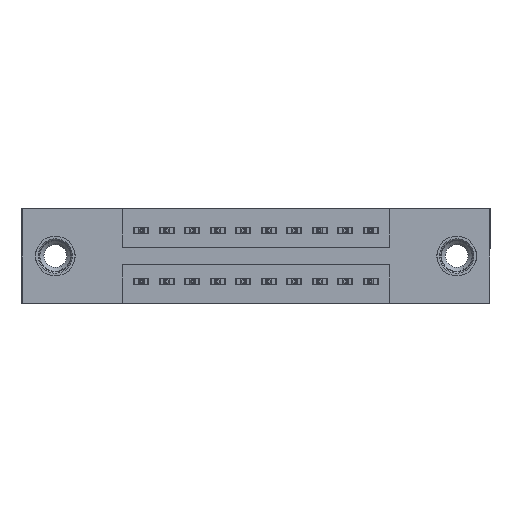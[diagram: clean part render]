
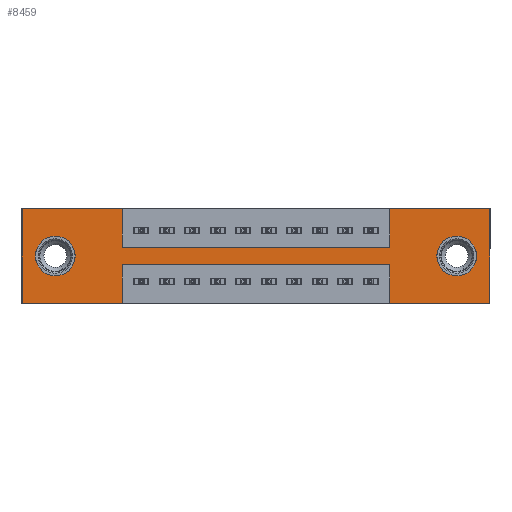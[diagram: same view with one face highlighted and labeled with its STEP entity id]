
A CAD part, front view. The second image highlights one B-rep face of the part: STEP entity #8459.
In plain terms, the highlighted planar face has unit normal (0, -1, 0).
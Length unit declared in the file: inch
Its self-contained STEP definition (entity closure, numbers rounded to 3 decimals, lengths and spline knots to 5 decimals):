
#154 = EDGE_CURVE ( 'NONE', #3749, #6685, #15151, .T. ) ;
#353 = LINE ( 'NONE', #451, #10246 ) ;
#451 = CARTESIAN_POINT ( 'NONE',  ( 0., 0., 0. ) ) ;
#562 = FACE_BOUND ( 'NONE', #4625, .T. ) ;
#708 = CARTESIAN_POINT ( 'NONE',  ( 0.3925, 0., 0. ) ) ;
#843 = ORIENTED_EDGE ( 'NONE', *, *, #6439, .T. ) ;
#929 = CARTESIAN_POINT ( 'NONE',  ( 1.4425, 0., -0.37 ) ) ;
#1437 = CARTESIAN_POINT ( 'NONE',  ( 1.705, 0., -0.185 ) ) ;
#1445 = DIRECTION ( 'NONE',  ( 0., 0., -1. ) ) ;
#1516 = ORIENTED_EDGE ( 'NONE', *, *, #12163, .F. ) ;
#1528 = CIRCLE ( 'NONE', #5353, 0.078 ) ;
#1596 = ORIENTED_EDGE ( 'NONE', *, *, #9845, .F. ) ;
#1669 = EDGE_CURVE ( 'NONE', #5775, #5150, #353, .T. ) ;
#1705 = CARTESIAN_POINT ( 'NONE',  ( 1.705, 0., -0.185 ) ) ;
#1790 = CARTESIAN_POINT ( 'NONE',  ( 0., 0., -0.37 ) ) ;
#1940 = VERTEX_POINT ( 'NONE', #9528 ) ;
#1948 = EDGE_CURVE ( 'NONE', #10972, #14394, #8327, .T. ) ;
#2037 = CIRCLE ( 'NONE', #12789, 0.078 ) ;
#3051 = CARTESIAN_POINT ( 'NONE',  ( 1.4425, 0., -0.15 ) ) ;
#3208 = PLANE ( 'NONE',  #11015 ) ;
#3228 = ORIENTED_EDGE ( 'NONE', *, *, #1948, .F. ) ;
#3576 = DIRECTION ( 'NONE',  ( 0., 0., 1. ) ) ;
#3749 = VERTEX_POINT ( 'NONE', #12784 ) ;
#3779 = CARTESIAN_POINT ( 'NONE',  ( 0., 0., 0. ) ) ;
#3935 = VECTOR ( 'NONE', #9086, 39.37008 ) ;
#4099 = DIRECTION ( 'NONE',  ( 0., 1., 0. ) ) ;
#4130 = VERTEX_POINT ( 'NONE', #3051 ) ;
#4337 = FACE_BOUND ( 'NONE', #5839, .T. ) ;
#4475 = VECTOR ( 'NONE', #3576, 39.37008 ) ;
#4580 = EDGE_CURVE ( 'NONE', #4130, #15901, #7280, .T. ) ;
#4591 = DIRECTION ( 'NONE',  ( 0., 0., -1. ) ) ;
#4625 = EDGE_LOOP ( 'NONE', ( #10248, #14746 ) ) ;
#4669 = ORIENTED_EDGE ( 'NONE', *, *, #7293, .F. ) ;
#4814 = AXIS2_PLACEMENT_3D ( 'NONE', #14560, #11875, #7838 ) ;
#5031 = LINE ( 'NONE', #10296, #3935 ) ;
#5150 = VERTEX_POINT ( 'NONE', #14241 ) ;
#5263 = ORIENTED_EDGE ( 'NONE', *, *, #4580, .F. ) ;
#5353 = AXIS2_PLACEMENT_3D ( 'NONE', #12979, #8852, #14101 ) ;
#5396 = ORIENTED_EDGE ( 'NONE', *, *, #13739, .F. ) ;
#5527 = VERTEX_POINT ( 'NONE', #10164 ) ;
#5775 = VERTEX_POINT ( 'NONE', #10461 ) ;
#5839 = EDGE_LOOP ( 'NONE', ( #843, #9866 ) ) ;
#5891 = DIRECTION ( 'NONE',  ( 1., 0., 0. ) ) ;
#5895 = CARTESIAN_POINT ( 'NONE',  ( 0., 0., -0.37 ) ) ;
#6199 = CARTESIAN_POINT ( 'NONE',  ( 0.3925, 0., -0.22 ) ) ;
#6439 = EDGE_CURVE ( 'NONE', #14237, #13422, #1528, .T. ) ;
#6487 = CARTESIAN_POINT ( 'NONE',  ( 1.835, 0., -0.37 ) ) ;
#6685 = VERTEX_POINT ( 'NONE', #11771 ) ;
#7280 = LINE ( 'NONE', #16972, #16041 ) ;
#7293 = EDGE_CURVE ( 'NONE', #1940, #15609, #16940, .T. ) ;
#7363 = CARTESIAN_POINT ( 'NONE',  ( 1.835, 0., 0. ) ) ;
#7439 = ORIENTED_EDGE ( 'NONE', *, *, #16641, .F. ) ;
#7478 = VECTOR ( 'NONE', #16711, 39.37008 ) ;
#7573 = VECTOR ( 'NONE', #12430, 39.37008 ) ;
#7838 = DIRECTION ( 'NONE',  ( 0., 0., 1. ) ) ;
#7875 = CARTESIAN_POINT ( 'NONE',  ( 0., 0., 0. ) ) ;
#8327 = LINE ( 'NONE', #1790, #8622 ) ;
#8349 = ORIENTED_EDGE ( 'NONE', *, *, #14571, .F. ) ;
#8449 = LINE ( 'NONE', #15230, #16773 ) ;
#8459 = ADVANCED_FACE ( 'NONE', ( #562, #4337, #9596 ), #3208, .T. ) ;
#8622 = VECTOR ( 'NONE', #13603, 39.37008 ) ;
#8785 = CARTESIAN_POINT ( 'NONE',  ( 0.13, 0., -0.263 ) ) ;
#8852 = DIRECTION ( 'NONE',  ( 0., 1., 0. ) ) ;
#8982 = ORIENTED_EDGE ( 'NONE', *, *, #16790, .F. ) ;
#9003 = EDGE_CURVE ( 'NONE', #6685, #3749, #2037, .T. ) ;
#9086 = DIRECTION ( 'NONE',  ( -1., 0., 0. ) ) ;
#9260 = ORIENTED_EDGE ( 'NONE', *, *, #1669, .F. ) ;
#9350 = DIRECTION ( 'NONE',  ( 0., 1., 0. ) ) ;
#9438 = VECTOR ( 'NONE', #5891, 39.37008 ) ;
#9490 = EDGE_CURVE ( 'NONE', #11828, #5775, #5031, .T. ) ;
#9528 = CARTESIAN_POINT ( 'NONE',  ( 1.4425, 0., -0.22 ) ) ;
#9596 = FACE_OUTER_BOUND ( 'NONE', #16831, .T. ) ;
#9715 = ORIENTED_EDGE ( 'NONE', *, *, #9490, .F. ) ;
#9831 = VECTOR ( 'NONE', #14142, 39.37008 ) ;
#9845 = EDGE_CURVE ( 'NONE', #15901, #14281, #10275, .T. ) ;
#9866 = ORIENTED_EDGE ( 'NONE', *, *, #16943, .T. ) ;
#9953 = CARTESIAN_POINT ( 'NONE',  ( 1.835, 0., 0. ) ) ;
#10164 = CARTESIAN_POINT ( 'NONE',  ( 0.3925, 0., -0.15 ) ) ;
#10167 = CARTESIAN_POINT ( 'NONE',  ( 0.3925, 0., -0.22 ) ) ;
#10246 = VECTOR ( 'NONE', #10674, 39.37008 ) ;
#10248 = ORIENTED_EDGE ( 'NONE', *, *, #9003, .T. ) ;
#10275 = LINE ( 'NONE', #3779, #7478 ) ;
#10296 = CARTESIAN_POINT ( 'NONE',  ( 0., 0., -0.37 ) ) ;
#10461 = CARTESIAN_POINT ( 'NONE',  ( 0., 0., -0.37 ) ) ;
#10674 = DIRECTION ( 'NONE',  ( 0., 0., 1. ) ) ;
#10785 = VECTOR ( 'NONE', #15373, 39.37008 ) ;
#10972 = VERTEX_POINT ( 'NONE', #6487 ) ;
#11015 = AXIS2_PLACEMENT_3D ( 'NONE', #5895, #12463, #4591 ) ;
#11027 = AXIS2_PLACEMENT_3D ( 'NONE', #1437, #9350, #14619 ) ;
#11074 = LINE ( 'NONE', #9953, #10785 ) ;
#11574 = DIRECTION ( 'NONE',  ( 1., 0., 0. ) ) ;
#11696 = CIRCLE ( 'NONE', #4814, 0.078 ) ;
#11771 = CARTESIAN_POINT ( 'NONE',  ( 1.705, 0., -0.107 ) ) ;
#11786 = CARTESIAN_POINT ( 'NONE',  ( 0.3925, 0., -0.37 ) ) ;
#11796 = CARTESIAN_POINT ( 'NONE',  ( 1.4425, 0., -0.37 ) ) ;
#11828 = VERTEX_POINT ( 'NONE', #11786 ) ;
#11875 = DIRECTION ( 'NONE',  ( 0., 1., 0. ) ) ;
#11923 = LINE ( 'NONE', #708, #7573 ) ;
#12023 = ORIENTED_EDGE ( 'NONE', *, *, #14243, .F. ) ;
#12163 = EDGE_CURVE ( 'NONE', #15609, #11828, #8449, .T. ) ;
#12430 = DIRECTION ( 'NONE',  ( 0., 0., -1. ) ) ;
#12463 = DIRECTION ( 'NONE',  ( 0., -1., 0. ) ) ;
#12662 = DIRECTION ( 'NONE',  ( 0., 0., -1. ) ) ;
#12784 = CARTESIAN_POINT ( 'NONE',  ( 1.705, 0., -0.263 ) ) ;
#12789 = AXIS2_PLACEMENT_3D ( 'NONE', #1705, #4099, #1445 ) ;
#12885 = DIRECTION ( 'NONE',  ( 0., 0., 1. ) ) ;
#12979 = CARTESIAN_POINT ( 'NONE',  ( 0.13, 0., -0.185 ) ) ;
#13422 = VERTEX_POINT ( 'NONE', #8785 ) ;
#13603 = DIRECTION ( 'NONE',  ( -1., 0., 0. ) ) ;
#13636 = LINE ( 'NONE', #929, #4475 ) ;
#13657 = VECTOR ( 'NONE', #11574, 39.37008 ) ;
#13739 = EDGE_CURVE ( 'NONE', #14281, #10972, #11074, .T. ) ;
#13877 = CARTESIAN_POINT ( 'NONE',  ( 0.3925, 0., 0. ) ) ;
#14101 = DIRECTION ( 'NONE',  ( 0., 0., 1. ) ) ;
#14142 = DIRECTION ( 'NONE',  ( -1., 0., 0. ) ) ;
#14237 = VERTEX_POINT ( 'NONE', #16465 ) ;
#14241 = CARTESIAN_POINT ( 'NONE',  ( 0., 0., 0. ) ) ;
#14243 = EDGE_CURVE ( 'NONE', #5527, #4130, #16541, .T. ) ;
#14281 = VERTEX_POINT ( 'NONE', #7363 ) ;
#14394 = VERTEX_POINT ( 'NONE', #11796 ) ;
#14560 = CARTESIAN_POINT ( 'NONE',  ( 0.13, 0., -0.185 ) ) ;
#14571 = EDGE_CURVE ( 'NONE', #14394, #1940, #13636, .T. ) ;
#14619 = DIRECTION ( 'NONE',  ( 0., 0., -1. ) ) ;
#14670 = VERTEX_POINT ( 'NONE', #13877 ) ;
#14746 = ORIENTED_EDGE ( 'NONE', *, *, #154, .T. ) ;
#15106 = CARTESIAN_POINT ( 'NONE',  ( 0.3925, 0., -0.15 ) ) ;
#15151 = CIRCLE ( 'NONE', #11027, 0.078 ) ;
#15230 = CARTESIAN_POINT ( 'NONE',  ( 0.3925, 0., -0.37 ) ) ;
#15373 = DIRECTION ( 'NONE',  ( 0., 0., -1. ) ) ;
#15448 = LINE ( 'NONE', #7875, #13657 ) ;
#15609 = VERTEX_POINT ( 'NONE', #6199 ) ;
#15901 = VERTEX_POINT ( 'NONE', #16170 ) ;
#16041 = VECTOR ( 'NONE', #12885, 39.37008 ) ;
#16170 = CARTESIAN_POINT ( 'NONE',  ( 1.4425, 0., 0. ) ) ;
#16465 = CARTESIAN_POINT ( 'NONE',  ( 0.13, 0., -0.107 ) ) ;
#16541 = LINE ( 'NONE', #15106, #9438 ) ;
#16641 = EDGE_CURVE ( 'NONE', #5150, #14670, #15448, .T. ) ;
#16711 = DIRECTION ( 'NONE',  ( 1., 0., 0. ) ) ;
#16773 = VECTOR ( 'NONE', #12662, 39.37008 ) ;
#16790 = EDGE_CURVE ( 'NONE', #14670, #5527, #11923, .T. ) ;
#16831 = EDGE_LOOP ( 'NONE', ( #1516, #4669, #8349, #3228, #5396, #1596, #5263, #12023, #8982, #7439, #9260, #9715 ) ) ;
#16940 = LINE ( 'NONE', #10167, #9831 ) ;
#16943 = EDGE_CURVE ( 'NONE', #13422, #14237, #11696, .T. ) ;
#16972 = CARTESIAN_POINT ( 'NONE',  ( 1.4425, 0., 0. ) ) ;
